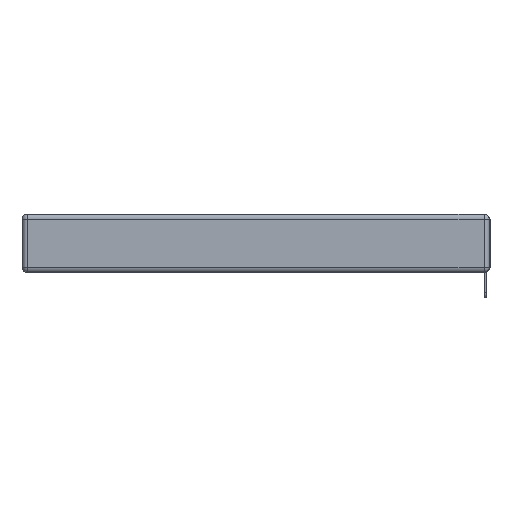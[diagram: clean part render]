
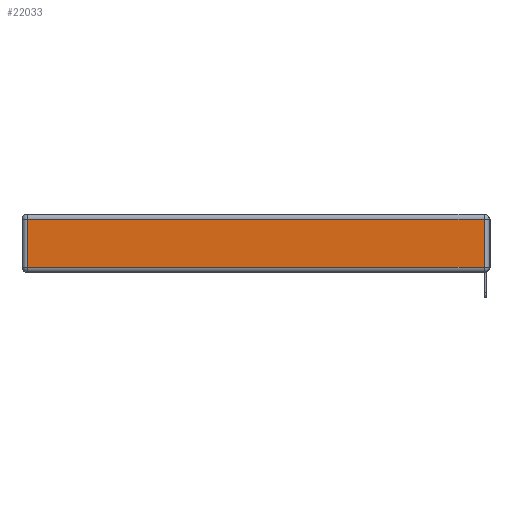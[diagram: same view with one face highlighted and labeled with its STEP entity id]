
A CAD part, left-side view. The second image highlights one B-rep face of the part: STEP entity #22033.
In plain terms, the highlighted planar face has unit normal (-1, 0, 0).
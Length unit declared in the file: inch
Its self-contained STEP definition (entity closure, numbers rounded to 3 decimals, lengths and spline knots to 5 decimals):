
#4573 = DIRECTION ( 'NONE',  ( 0., 1., 0. ) ) ;
#5679 = EDGE_CURVE ( 'NONE', #14952, #13173, #21884, .T. ) ;
#6517 = FACE_OUTER_BOUND ( 'NONE', #21559, .T. ) ;
#6636 = DIRECTION ( 'NONE',  ( 0., 0., 1. ) ) ;
#7450 = ORIENTED_EDGE ( 'NONE', *, *, #5679, .T. ) ;
#8409 = CARTESIAN_POINT ( 'NONE',  ( 0., 0., -0.343 ) ) ;
#8440 = CARTESIAN_POINT ( 'NONE',  ( 0., 0., -0.313 ) ) ;
#8930 = ORIENTED_EDGE ( 'NONE', *, *, #13830, .T. ) ;
#10609 = VERTEX_POINT ( 'NONE', #15764 ) ;
#11275 = CARTESIAN_POINT ( 'NONE',  ( 0., 2.72, -0.343 ) ) ;
#11568 = CARTESIAN_POINT ( 'NONE',  ( 0., 2.72, -0.313 ) ) ;
#12955 = DIRECTION ( 'NONE',  ( 0., 0., -1. ) ) ;
#13075 = VECTOR ( 'NONE', #22521, 39.37008 ) ;
#13173 = VERTEX_POINT ( 'NONE', #11568 ) ;
#13532 = CARTESIAN_POINT ( 'NONE',  ( 0., 2.75, -0.03 ) ) ;
#13803 = VECTOR ( 'NONE', #4573, 39.37008 ) ;
#13830 = EDGE_CURVE ( 'NONE', #10609, #23028, #14041, .T. ) ;
#14041 = LINE ( 'NONE', #23314, #20826 ) ;
#14952 = VERTEX_POINT ( 'NONE', #15038 ) ;
#15038 = CARTESIAN_POINT ( 'NONE',  ( 0., 2.72, -0.03 ) ) ;
#15764 = CARTESIAN_POINT ( 'NONE',  ( 0., 0.03, -0.313 ) ) ;
#15961 = DIRECTION ( 'NONE',  ( 0., 0., 1. ) ) ;
#16071 = PLANE ( 'NONE',  #18376 ) ;
#16797 = ORIENTED_EDGE ( 'NONE', *, *, #22278, .T. ) ;
#18376 = AXIS2_PLACEMENT_3D ( 'NONE', #8409, #21053, #6636 ) ;
#18933 = ORIENTED_EDGE ( 'NONE', *, *, #22603, .T. ) ;
#20826 = VECTOR ( 'NONE', #15961, 39.37008 ) ;
#21053 = DIRECTION ( 'NONE',  ( -1., 0., 0. ) ) ;
#21081 = LINE ( 'NONE', #8440, #13075 ) ;
#21559 = EDGE_LOOP ( 'NONE', ( #18933, #8930, #16797, #7450 ) ) ;
#21884 = LINE ( 'NONE', #11275, #22898 ) ;
#22033 = ADVANCED_FACE ( 'NONE', ( #6517 ), #16071, .T. ) ;
#22278 = EDGE_CURVE ( 'NONE', #23028, #14952, #22578, .T. ) ;
#22521 = DIRECTION ( 'NONE',  ( 0., -1., 0. ) ) ;
#22578 = LINE ( 'NONE', #13532, #13803 ) ;
#22603 = EDGE_CURVE ( 'NONE', #13173, #10609, #21081, .T. ) ;
#22688 = CARTESIAN_POINT ( 'NONE',  ( 0., 0.03, -0.03 ) ) ;
#22898 = VECTOR ( 'NONE', #12955, 39.37008 ) ;
#23028 = VERTEX_POINT ( 'NONE', #22688 ) ;
#23314 = CARTESIAN_POINT ( 'NONE',  ( 0., 0.03, -0.343 ) ) ;
